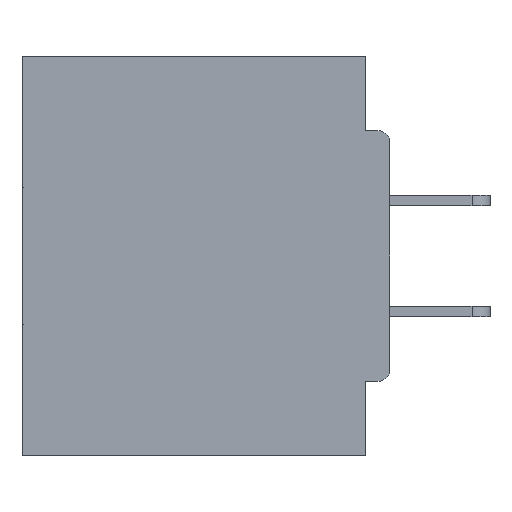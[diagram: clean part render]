
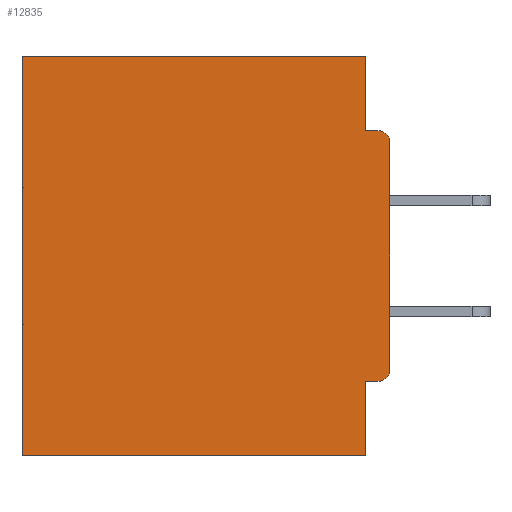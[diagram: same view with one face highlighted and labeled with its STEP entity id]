
A CAD part, left-side view. The second image highlights one B-rep face of the part: STEP entity #12835.
In plain terms, the highlighted planar face has unit normal (-1, 0, 0).
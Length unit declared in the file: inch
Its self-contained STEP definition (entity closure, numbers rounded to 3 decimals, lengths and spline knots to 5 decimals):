
#195 = LINE ( 'NONE', #24741, #3893 ) ;
#401 = VERTEX_POINT ( 'NONE', #38901 ) ;
#426 = ORIENTED_EDGE ( 'NONE', *, *, #14787, .T. ) ;
#2203 = ORIENTED_EDGE ( 'NONE', *, *, #5922, .T. ) ;
#2668 = LINE ( 'NONE', #41041, #41002 ) ;
#2754 = EDGE_CURVE ( 'NONE', #6542, #27602, #195, .T. ) ;
#2988 = VECTOR ( 'NONE', #12026, 39.37008 ) ;
#3893 = VECTOR ( 'NONE', #8831, 39.37008 ) ;
#4079 = ORIENTED_EDGE ( 'NONE', *, *, #25840, .F. ) ;
#4145 = CARTESIAN_POINT ( 'NONE',  ( 0.298, 0.031, -0.5 ) ) ;
#4247 = CARTESIAN_POINT ( 'NONE',  ( 0.298, 0.015, -0.3915 ) ) ;
#4513 = DIRECTION ( 'NONE',  ( -1., 0., 0. ) ) ;
#5080 = CARTESIAN_POINT ( 'NONE',  ( 0.298, 0., 0. ) ) ;
#5502 = DIRECTION ( 'NONE',  ( 0., 0., -1. ) ) ;
#5922 = EDGE_CURVE ( 'NONE', #401, #19792, #38004, .T. ) ;
#6318 = CARTESIAN_POINT ( 'NONE',  ( 0.298, 0.015, -0.0935 ) ) ;
#6419 = EDGE_CURVE ( 'NONE', #28808, #19792, #31490, .T. ) ;
#6542 = VERTEX_POINT ( 'NONE', #14236 ) ;
#7379 = EDGE_CURVE ( 'NONE', #22822, #23879, #21027, .T. ) ;
#7567 = EDGE_CURVE ( 'NONE', #38478, #6542, #23496, .T. ) ;
#7731 = DIRECTION ( 'NONE',  ( 0., 0., -1. ) ) ;
#8127 = DIRECTION ( 'NONE',  ( 0., 1., 0. ) ) ;
#8831 = DIRECTION ( 'NONE',  ( 0., -1., 0. ) ) ;
#9494 = ORIENTED_EDGE ( 'NONE', *, *, #28702, .T. ) ;
#10888 = FACE_OUTER_BOUND ( 'NONE', #12287, .T. ) ;
#12026 = DIRECTION ( 'NONE',  ( 0., 0., -1. ) ) ;
#12192 = DIRECTION ( 'NONE',  ( -1., 0., 0. ) ) ;
#12287 = EDGE_LOOP ( 'NONE', ( #9494, #37837, #31291, #23240, #426, #24727, #34476, #4079, #2203, #29085 ) ) ;
#12402 = AXIS2_PLACEMENT_3D ( 'NONE', #4247, #4513, #7731 ) ;
#12835 = ADVANCED_FACE ( 'NONE', ( #10888 ), #35048, .F. ) ;
#13678 = CARTESIAN_POINT ( 'NONE',  ( 0.298, 0.031, -0.5 ) ) ;
#14236 = CARTESIAN_POINT ( 'NONE',  ( 0.298, 0.031, -0.0935 ) ) ;
#14787 = EDGE_CURVE ( 'NONE', #21561, #18797, #2668, .T. ) ;
#14806 = CIRCLE ( 'NONE', #33042, 0.015 ) ;
#16046 = EDGE_CURVE ( 'NONE', #23879, #18797, #36545, .T. ) ;
#16826 = LINE ( 'NONE', #33327, #33668 ) ;
#18797 = VERTEX_POINT ( 'NONE', #28997 ) ;
#19721 = CARTESIAN_POINT ( 'NONE',  ( 0.298, 0., 0. ) ) ;
#19792 = VERTEX_POINT ( 'NONE', #39018 ) ;
#19941 = EDGE_CURVE ( 'NONE', #38478, #21561, #35765, .T. ) ;
#20337 = DIRECTION ( 'NONE',  ( 0., 1., 0. ) ) ;
#21027 = LINE ( 'NONE', #41048, #2988 ) ;
#21561 = VERTEX_POINT ( 'NONE', #35140 ) ;
#22616 = DIRECTION ( 'NONE',  ( 1., 0., 0. ) ) ;
#22822 = VERTEX_POINT ( 'NONE', #30312 ) ;
#23182 = DIRECTION ( 'NONE',  ( 0., 0., -1. ) ) ;
#23240 = ORIENTED_EDGE ( 'NONE', *, *, #19941, .T. ) ;
#23412 = VECTOR ( 'NONE', #35199, 39.37008 ) ;
#23496 = LINE ( 'NONE', #13678, #28911 ) ;
#23879 = VERTEX_POINT ( 'NONE', #4145 ) ;
#24727 = ORIENTED_EDGE ( 'NONE', *, *, #16046, .F. ) ;
#24741 = CARTESIAN_POINT ( 'NONE',  ( 0.298, 0., -0.0935 ) ) ;
#25538 = DIRECTION ( 'NONE',  ( 0., 0., -1. ) ) ;
#25840 = EDGE_CURVE ( 'NONE', #401, #22822, #16826, .T. ) ;
#27078 = CARTESIAN_POINT ( 'NONE',  ( 0.298, 0., -0.5 ) ) ;
#27602 = VERTEX_POINT ( 'NONE', #6318 ) ;
#28141 = VECTOR ( 'NONE', #8127, 39.37008 ) ;
#28702 = EDGE_CURVE ( 'NONE', #28808, #27602, #14806, .T. ) ;
#28808 = VERTEX_POINT ( 'NONE', #34534 ) ;
#28911 = VECTOR ( 'NONE', #29257, 39.37008 ) ;
#28997 = CARTESIAN_POINT ( 'NONE',  ( 0.298, 0.46, -0.5 ) ) ;
#29085 = ORIENTED_EDGE ( 'NONE', *, *, #6419, .F. ) ;
#29257 = DIRECTION ( 'NONE',  ( 0., 0., -1. ) ) ;
#30312 = CARTESIAN_POINT ( 'NONE',  ( 0.298, 0.031, -0.4065 ) ) ;
#31291 = ORIENTED_EDGE ( 'NONE', *, *, #7567, .F. ) ;
#31490 = LINE ( 'NONE', #19721, #36442 ) ;
#32166 = DIRECTION ( 'NONE',  ( 0., 0., -1. ) ) ;
#33042 = AXIS2_PLACEMENT_3D ( 'NONE', #37297, #12192, #5502 ) ;
#33327 = CARTESIAN_POINT ( 'NONE',  ( 0.298, 0., -0.4065 ) ) ;
#33668 = VECTOR ( 'NONE', #20337, 39.37008 ) ;
#34476 = ORIENTED_EDGE ( 'NONE', *, *, #7379, .F. ) ;
#34534 = CARTESIAN_POINT ( 'NONE',  ( 0.298, 0., -0.1085 ) ) ;
#35048 = PLANE ( 'NONE',  #41033 ) ;
#35140 = CARTESIAN_POINT ( 'NONE',  ( 0.298, 0.46, 0. ) ) ;
#35199 = DIRECTION ( 'NONE',  ( 0., 1., 0. ) ) ;
#35319 = CARTESIAN_POINT ( 'NONE',  ( 0.298, 0., 0. ) ) ;
#35765 = LINE ( 'NONE', #5080, #23412 ) ;
#36442 = VECTOR ( 'NONE', #32166, 39.37008 ) ;
#36545 = LINE ( 'NONE', #27078, #28141 ) ;
#37297 = CARTESIAN_POINT ( 'NONE',  ( 0.298, 0.015, -0.1085 ) ) ;
#37837 = ORIENTED_EDGE ( 'NONE', *, *, #2754, .F. ) ;
#38004 = CIRCLE ( 'NONE', #12402, 0.015 ) ;
#38478 = VERTEX_POINT ( 'NONE', #40772 ) ;
#38901 = CARTESIAN_POINT ( 'NONE',  ( 0.298, 0.015, -0.4065 ) ) ;
#39018 = CARTESIAN_POINT ( 'NONE',  ( 0.298, 0., -0.3915 ) ) ;
#40772 = CARTESIAN_POINT ( 'NONE',  ( 0.298, 0.031, 0. ) ) ;
#41002 = VECTOR ( 'NONE', #23182, 39.37008 ) ;
#41033 = AXIS2_PLACEMENT_3D ( 'NONE', #35319, #22616, #25538 ) ;
#41041 = CARTESIAN_POINT ( 'NONE',  ( 0.298, 0.46, 0. ) ) ;
#41048 = CARTESIAN_POINT ( 'NONE',  ( 0.298, 0.031, -0.5 ) ) ;
